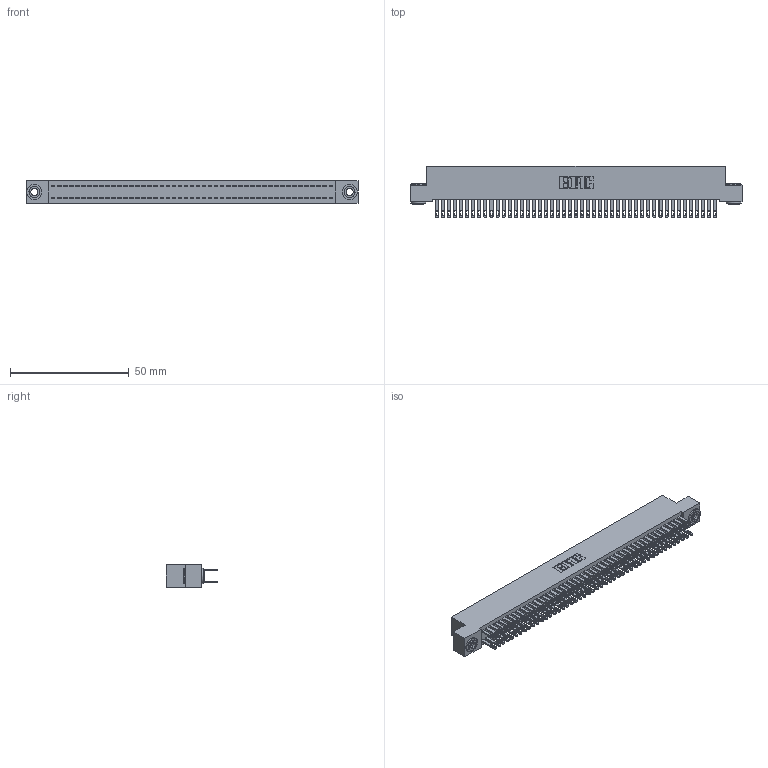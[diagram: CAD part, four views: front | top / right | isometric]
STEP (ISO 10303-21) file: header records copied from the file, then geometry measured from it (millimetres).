
FILE_DESCRIPTION (( 'STEP AP203' ), '1' );
FILE_NAME ('342-094-500-203.STEP', '2018-08-14T02:13:50', ( '' ), ( '' ), 'SwSTEP 2.0', 'SolidWorks 2016', '' );
FILE_SCHEMA (( 'CONFIG_CONTROL_DESIGN' ));
Length unit declared in the file: inch
Products named in the file (4): 342-250-002_345-250-002-102; 342-094-500-203; 342 Part_.156 TH; 345-292-001_345-293-100
Assembly tree (97 placements, depth 2):
  342-094-500-203
    342 Part_.156 TH
    345-292-001_345-293-100  x94
    342-250-002_345-250-002-102  x2
Bounding box: 139.7 x 21.85 x 9.4 mm (x, y, z)
Volume: 12885.8 mm3; surface area: 22212.1 mm2
Topology: 97 solids, 97 shells, 4660 faces, 14193 edges, 9458 vertices
Faces by surface type: plane 2896, cylinder 1756, cone 8
Entity records: 30038 total; most frequent: CARTESIAN_POINT 4945, ORIENTED_EDGE 4874, DIRECTION 4251, EDGE_CURVE 2437, VECTOR 2281, LINE 2281, VERTEX_POINT 1622, AXIS2_PLACEMENT_3D 985
